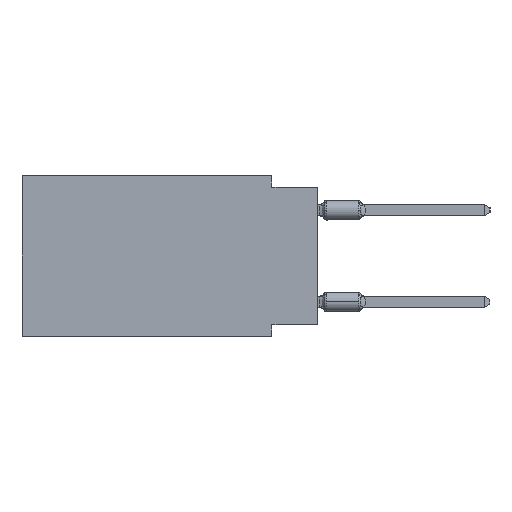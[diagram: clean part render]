
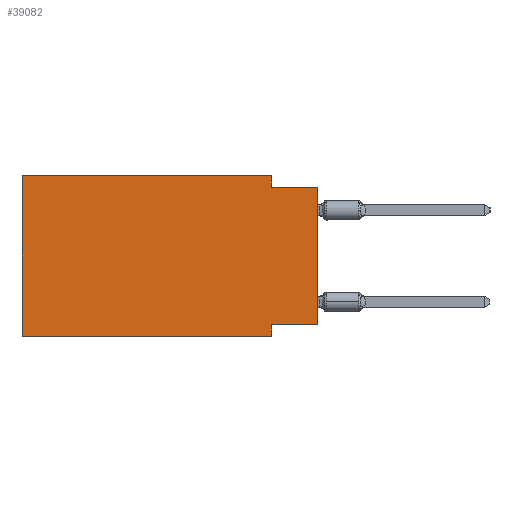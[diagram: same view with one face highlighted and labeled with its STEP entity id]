
A CAD part, left-side view. The second image highlights one B-rep face of the part: STEP entity #39082.
In plain terms, the highlighted planar face has unit normal (-1, 0, 0).
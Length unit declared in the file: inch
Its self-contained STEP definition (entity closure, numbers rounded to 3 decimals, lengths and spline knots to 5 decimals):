
#168 = EDGE_CURVE ( 'NONE', #34881, #884, #10197, .T. ) ;
#233 = CARTESIAN_POINT ( 'NONE',  ( 0., 0.1, -0.35 ) ) ;
#263 = CARTESIAN_POINT ( 'NONE',  ( 0., 0.1, 0. ) ) ;
#884 = VERTEX_POINT ( 'NONE', #36465 ) ;
#1344 = VECTOR ( 'NONE', #13643, 39.37008 ) ;
#2396 = VECTOR ( 'NONE', #19552, 39.37008 ) ;
#3100 = VECTOR ( 'NONE', #9054, 39.37008 ) ;
#4574 = VERTEX_POINT ( 'NONE', #35670 ) ;
#7725 = VERTEX_POINT ( 'NONE', #16238 ) ;
#7761 = LINE ( 'NONE', #233, #2396 ) ;
#8338 = DIRECTION ( 'NONE',  ( 0., 0., -1. ) ) ;
#8458 = DIRECTION ( 'NONE',  ( 0., -1., 0. ) ) ;
#9054 = DIRECTION ( 'NONE',  ( 0., 0., 1. ) ) ;
#9212 = CARTESIAN_POINT ( 'NONE',  ( 0., 0., -0.325 ) ) ;
#9422 = DIRECTION ( 'NONE',  ( 0., 0., 1. ) ) ;
#9712 = LINE ( 'NONE', #9212, #18464 ) ;
#10197 = LINE ( 'NONE', #33194, #41341 ) ;
#11196 = VERTEX_POINT ( 'NONE', #47259 ) ;
#13643 = DIRECTION ( 'NONE',  ( 0., -1., 0. ) ) ;
#13793 = EDGE_CURVE ( 'NONE', #31035, #4574, #39914, .T. ) ;
#13807 = CARTESIAN_POINT ( 'NONE',  ( 0., 0.645, -0.35 ) ) ;
#16238 = CARTESIAN_POINT ( 'NONE',  ( 0., 0., -0.325 ) ) ;
#16269 = ORIENTED_EDGE ( 'NONE', *, *, #13793, .F. ) ;
#16576 = CARTESIAN_POINT ( 'NONE',  ( 0., 0.645, -0.35 ) ) ;
#16946 = FACE_OUTER_BOUND ( 'NONE', #45881, .T. ) ;
#17054 = LINE ( 'NONE', #29066, #1344 ) ;
#17101 = VERTEX_POINT ( 'NONE', #36017 ) ;
#17340 = ORIENTED_EDGE ( 'NONE', *, *, #38162, .F. ) ;
#18464 = VECTOR ( 'NONE', #25131, 39.37008 ) ;
#19552 = DIRECTION ( 'NONE',  ( 0., 0., -1. ) ) ;
#19978 = VERTEX_POINT ( 'NONE', #33050 ) ;
#20478 = LINE ( 'NONE', #23883, #23579 ) ;
#22047 = VECTOR ( 'NONE', #8338, 39.37008 ) ;
#23579 = VECTOR ( 'NONE', #47856, 39.37008 ) ;
#23883 = CARTESIAN_POINT ( 'NONE',  ( 0., 0., -0.025 ) ) ;
#24229 = CARTESIAN_POINT ( 'NONE',  ( 0., 0.1, 0. ) ) ;
#25131 = DIRECTION ( 'NONE',  ( 0., 1., 0. ) ) ;
#27722 = EDGE_CURVE ( 'NONE', #19978, #11196, #7761, .T. ) ;
#27848 = ORIENTED_EDGE ( 'NONE', *, *, #27722, .F. ) ;
#28315 = ORIENTED_EDGE ( 'NONE', *, *, #40736, .F. ) ;
#29066 = CARTESIAN_POINT ( 'NONE',  ( 0., 0.645, 0. ) ) ;
#30367 = AXIS2_PLACEMENT_3D ( 'NONE', #49504, #32613, #32864 ) ;
#31035 = VERTEX_POINT ( 'NONE', #24229 ) ;
#32613 = DIRECTION ( 'NONE',  ( 1., 0., 0. ) ) ;
#32795 = LINE ( 'NONE', #48678, #3100 ) ;
#32864 = DIRECTION ( 'NONE',  ( 0., 0., -1. ) ) ;
#33050 = CARTESIAN_POINT ( 'NONE',  ( 0., 0.1, -0.325 ) ) ;
#33194 = CARTESIAN_POINT ( 'NONE',  ( 0., 0.645, 0. ) ) ;
#33966 = ORIENTED_EDGE ( 'NONE', *, *, #38077, .T. ) ;
#34881 = VERTEX_POINT ( 'NONE', #13807 ) ;
#35670 = CARTESIAN_POINT ( 'NONE',  ( 0., 0.1, -0.025 ) ) ;
#35720 = ORIENTED_EDGE ( 'NONE', *, *, #168, .F. ) ;
#36017 = CARTESIAN_POINT ( 'NONE',  ( 0., 0., -0.025 ) ) ;
#36465 = CARTESIAN_POINT ( 'NONE',  ( 0., 0.645, 0. ) ) ;
#38077 = EDGE_CURVE ( 'NONE', #34881, #11196, #51518, .T. ) ;
#38162 = EDGE_CURVE ( 'NONE', #4574, #17101, #20478, .T. ) ;
#39082 = ADVANCED_FACE ( 'NONE', ( #16946 ), #44843, .F. ) ;
#39914 = LINE ( 'NONE', #263, #22047 ) ;
#40736 = EDGE_CURVE ( 'NONE', #884, #31035, #17054, .T. ) ;
#41341 = VECTOR ( 'NONE', #9422, 39.37008 ) ;
#42068 = EDGE_CURVE ( 'NONE', #7725, #17101, #32795, .T. ) ;
#43464 = ORIENTED_EDGE ( 'NONE', *, *, #46207, .F. ) ;
#43587 = ORIENTED_EDGE ( 'NONE', *, *, #42068, .T. ) ;
#44843 = PLANE ( 'NONE',  #30367 ) ;
#45881 = EDGE_LOOP ( 'NONE', ( #43587, #17340, #16269, #28315, #35720, #33966, #27848, #43464 ) ) ;
#46207 = EDGE_CURVE ( 'NONE', #7725, #19978, #9712, .T. ) ;
#47259 = CARTESIAN_POINT ( 'NONE',  ( 0., 0.1, -0.35 ) ) ;
#47856 = DIRECTION ( 'NONE',  ( 0., -1., 0. ) ) ;
#48678 = CARTESIAN_POINT ( 'NONE',  ( 0., 0., 0. ) ) ;
#49504 = CARTESIAN_POINT ( 'NONE',  ( 0., 0.645, 0. ) ) ;
#51039 = VECTOR ( 'NONE', #8458, 39.37008 ) ;
#51518 = LINE ( 'NONE', #16576, #51039 ) ;
